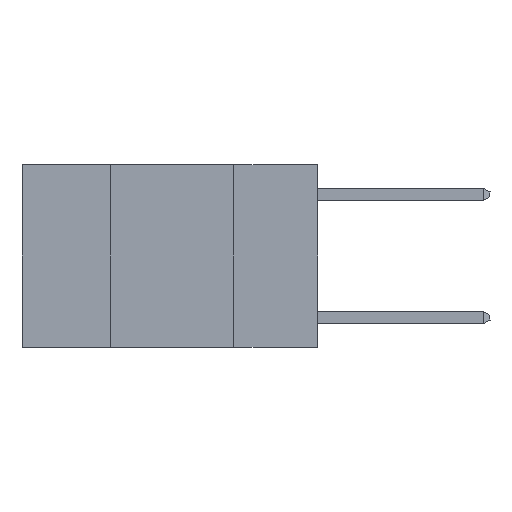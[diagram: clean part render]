
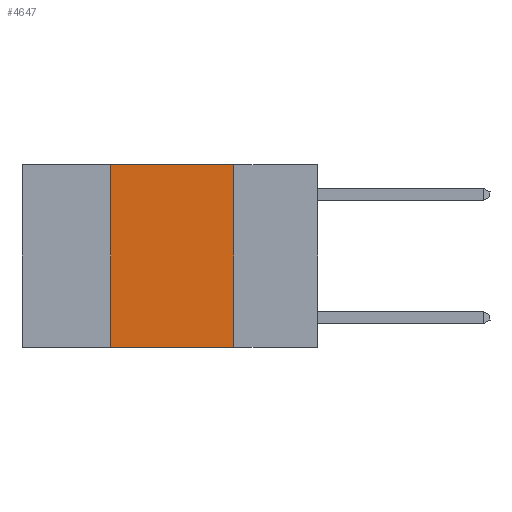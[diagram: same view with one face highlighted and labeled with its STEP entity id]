
A CAD part, left-side view. The second image highlights one B-rep face of the part: STEP entity #4647.
In plain terms, the highlighted planar face has unit normal (-1, 0, 0).
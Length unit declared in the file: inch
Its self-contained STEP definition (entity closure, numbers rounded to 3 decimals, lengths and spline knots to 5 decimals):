
#495 = DIRECTION ( 'NONE',  ( 0., -1., 0. ) ) ;
#590 = DIRECTION ( 'NONE',  ( 0., 0., -1. ) ) ;
#613 = LINE ( 'NONE', #12340, #18199 ) ;
#614 = ORIENTED_EDGE ( 'NONE', *, *, #21861, .F. ) ;
#1470 = DIRECTION ( 'NONE',  ( 1., 0., 0. ) ) ;
#1864 = DIRECTION ( 'NONE',  ( 0., -1., 0. ) ) ;
#3024 = EDGE_CURVE ( 'NONE', #5832, #20444, #5875, .T. ) ;
#3944 = ORIENTED_EDGE ( 'NONE', *, *, #11967, .T. ) ;
#4647 = ADVANCED_FACE ( 'NONE', ( #16946 ), #24533, .F. ) ;
#5493 = CARTESIAN_POINT ( 'NONE',  ( 0., 0.17, 0. ) ) ;
#5832 = VERTEX_POINT ( 'NONE', #5493 ) ;
#5875 = LINE ( 'NONE', #9729, #15332 ) ;
#6256 = VECTOR ( 'NONE', #16510, 39.37008 ) ;
#6683 = VERTEX_POINT ( 'NONE', #16516 ) ;
#7541 = AXIS2_PLACEMENT_3D ( 'NONE', #18559, #1470, #12047 ) ;
#9729 = CARTESIAN_POINT ( 'NONE',  ( 0., 0.17, 0. ) ) ;
#11447 = VECTOR ( 'NONE', #1864, 39.37008 ) ;
#11496 = CARTESIAN_POINT ( 'NONE',  ( 0., 0.42, 0. ) ) ;
#11841 = VERTEX_POINT ( 'NONE', #11496 ) ;
#11967 = EDGE_CURVE ( 'NONE', #6683, #20444, #13219, .T. ) ;
#12047 = DIRECTION ( 'NONE',  ( 0., 0., -1. ) ) ;
#12340 = CARTESIAN_POINT ( 'NONE',  ( 0., 0.6, 0. ) ) ;
#12765 = LINE ( 'NONE', #16266, #6256 ) ;
#13219 = LINE ( 'NONE', #20827, #11447 ) ;
#14523 = EDGE_CURVE ( 'NONE', #6683, #11841, #12765, .T. ) ;
#14785 = EDGE_LOOP ( 'NONE', ( #23386, #614, #17166, #3944 ) ) ;
#15332 = VECTOR ( 'NONE', #590, 39.37008 ) ;
#16137 = CARTESIAN_POINT ( 'NONE',  ( 0., 0.17, -0.37 ) ) ;
#16266 = CARTESIAN_POINT ( 'NONE',  ( 0., 0.42, 0. ) ) ;
#16510 = DIRECTION ( 'NONE',  ( 0., 0., 1. ) ) ;
#16516 = CARTESIAN_POINT ( 'NONE',  ( 0., 0.42, -0.37 ) ) ;
#16946 = FACE_OUTER_BOUND ( 'NONE', #14785, .T. ) ;
#17166 = ORIENTED_EDGE ( 'NONE', *, *, #14523, .F. ) ;
#18199 = VECTOR ( 'NONE', #495, 39.37008 ) ;
#18559 = CARTESIAN_POINT ( 'NONE',  ( 0., 0.6, 0. ) ) ;
#20444 = VERTEX_POINT ( 'NONE', #16137 ) ;
#20827 = CARTESIAN_POINT ( 'NONE',  ( 0., 0.6, -0.37 ) ) ;
#21861 = EDGE_CURVE ( 'NONE', #11841, #5832, #613, .T. ) ;
#23386 = ORIENTED_EDGE ( 'NONE', *, *, #3024, .F. ) ;
#24533 = PLANE ( 'NONE',  #7541 ) ;
